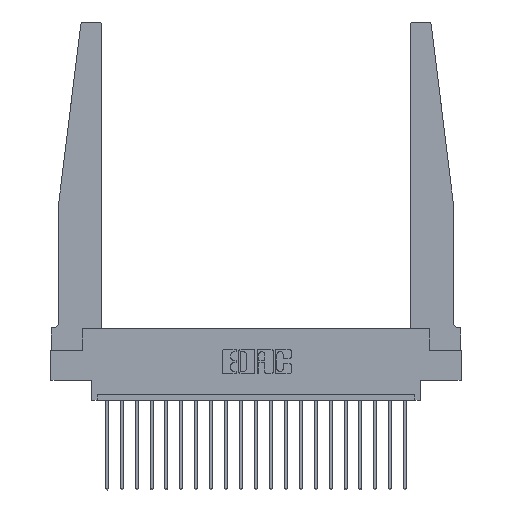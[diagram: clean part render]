
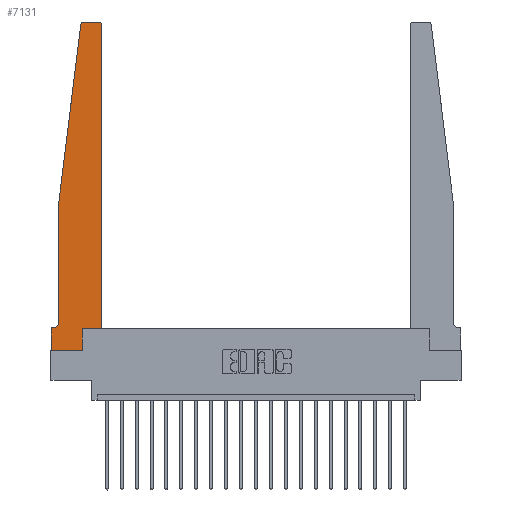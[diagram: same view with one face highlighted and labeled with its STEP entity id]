
A CAD part, top view. The second image highlights one B-rep face of the part: STEP entity #7131.
In plain terms, the highlighted planar face has unit normal (0, 0, 1).
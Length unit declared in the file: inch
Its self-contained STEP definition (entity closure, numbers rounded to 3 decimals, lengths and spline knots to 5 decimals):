
#42 = VECTOR ( 'NONE', #8179, 39.37008 ) ;
#329 = LINE ( 'NONE', #2886, #16862 ) ;
#640 = CARTESIAN_POINT ( 'NONE',  ( 0.27653, 2.75, 0.37 ) ) ;
#908 = CARTESIAN_POINT ( 'NONE',  ( 0.2605, 0.18, 0.37 ) ) ;
#1044 = ORIENTED_EDGE ( 'NONE', *, *, #4860, .T. ) ;
#1061 = DIRECTION ( 'NONE',  ( 0., 0., 1. ) ) ;
#1256 = VERTEX_POINT ( 'NONE', #11830 ) ;
#1284 = VERTEX_POINT ( 'NONE', #15466 ) ;
#1334 = DIRECTION ( 'NONE',  ( 0., 0., -1. ) ) ;
#1591 = CARTESIAN_POINT ( 'NONE',  ( 0.425, 0.18, 0.37 ) ) ;
#1922 = VECTOR ( 'NONE', #6121, 39.37008 ) ;
#2094 = CIRCLE ( 'NONE', #14696, 0.03 ) ;
#2648 = CARTESIAN_POINT ( 'NONE',  ( 0.395, 2.75, 0.37 ) ) ;
#2691 = DIRECTION ( 'NONE',  ( -1., 0., 0. ) ) ;
#2886 = CARTESIAN_POINT ( 'NONE',  ( 0.425, 0.18, 0.37 ) ) ;
#3394 = DIRECTION ( 'NONE',  ( 0., 0., 1. ) ) ;
#3483 = EDGE_CURVE ( 'NONE', #14115, #4005, #6902, .T. ) ;
#3516 = LINE ( 'NONE', #5672, #9023 ) ;
#3577 = FACE_OUTER_BOUND ( 'NONE', #15233, .T. ) ;
#4005 = VERTEX_POINT ( 'NONE', #640 ) ;
#4260 = DIRECTION ( 'NONE',  ( -1., 0., 0. ) ) ;
#4605 = EDGE_CURVE ( 'NONE', #6205, #5960, #329, .T. ) ;
#4860 = EDGE_CURVE ( 'NONE', #5960, #14115, #2094, .T. ) ;
#4876 = CARTESIAN_POINT ( 'NONE',  ( 0.27653, 2.72, 0.37 ) ) ;
#5551 = EDGE_CURVE ( 'NONE', #1284, #20755, #17089, .T. ) ;
#5671 = EDGE_CURVE ( 'NONE', #1256, #15966, #12101, .T. ) ;
#5672 = CARTESIAN_POINT ( 'NONE',  ( 0., 0., 0.37 ) ) ;
#5826 = EDGE_CURVE ( 'NONE', #4005, #1284, #11844, .T. ) ;
#5905 = ORIENTED_EDGE ( 'NONE', *, *, #5671, .T. ) ;
#5960 = VERTEX_POINT ( 'NONE', #11725 ) ;
#6121 = DIRECTION ( 'NONE',  ( 1., 0., 0. ) ) ;
#6205 = VERTEX_POINT ( 'NONE', #7276 ) ;
#6884 = DIRECTION ( 'NONE',  ( 0., 0., 1. ) ) ;
#6890 = DIRECTION ( 'NONE',  ( 0., 1., 0. ) ) ;
#6902 = LINE ( 'NONE', #16911, #10949 ) ;
#6997 = ORIENTED_EDGE ( 'NONE', *, *, #5551, .T. ) ;
#7131 = ADVANCED_FACE ( 'NONE', ( #3577 ), #10405, .T. ) ;
#7273 = CARTESIAN_POINT ( 'NONE',  ( 0.2605, 0., 0.37 ) ) ;
#7276 = CARTESIAN_POINT ( 'NONE',  ( 0.425, 0.18, 0.37 ) ) ;
#7565 = VECTOR ( 'NONE', #12845, 39.37008 ) ;
#7809 = EDGE_CURVE ( 'NONE', #20755, #13291, #15121, .T. ) ;
#8127 = CARTESIAN_POINT ( 'NONE',  ( 0.065, 1.25, 0.37 ) ) ;
#8179 = DIRECTION ( 'NONE',  ( -0.122, -0.992, 0. ) ) ;
#8331 = CARTESIAN_POINT ( 'NONE',  ( 0.065, 1.25, 0.37 ) ) ;
#9023 = VECTOR ( 'NONE', #12078, 39.37008 ) ;
#9513 = ORIENTED_EDGE ( 'NONE', *, *, #19324, .T. ) ;
#9873 = VERTEX_POINT ( 'NONE', #14425 ) ;
#10405 = PLANE ( 'NONE',  #18043 ) ;
#10487 = VECTOR ( 'NONE', #6890, 39.37008 ) ;
#10492 = LINE ( 'NONE', #17233, #17969 ) ;
#10684 = AXIS2_PLACEMENT_3D ( 'NONE', #4876, #3394, #11198 ) ;
#10885 = EDGE_CURVE ( 'NONE', #14520, #9873, #10492, .T. ) ;
#10949 = VECTOR ( 'NONE', #4260, 39.37008 ) ;
#11198 = DIRECTION ( 'NONE',  ( 1., 0., 0. ) ) ;
#11725 = CARTESIAN_POINT ( 'NONE',  ( 0.425, 2.72, 0.37 ) ) ;
#11830 = CARTESIAN_POINT ( 'NONE',  ( 0., 0., 0.37 ) ) ;
#11844 = CIRCLE ( 'NONE', #10684, 0.03 ) ;
#12078 = DIRECTION ( 'NONE',  ( 0., -1., 0. ) ) ;
#12101 = LINE ( 'NONE', #12699, #7565 ) ;
#12557 = DIRECTION ( 'NONE',  ( -1., 0., 0. ) ) ;
#12597 = VECTOR ( 'NONE', #14299, 39.37008 ) ;
#12699 = CARTESIAN_POINT ( 'NONE',  ( 0., 0., 0.37 ) ) ;
#12845 = DIRECTION ( 'NONE',  ( 1., 0., 0. ) ) ;
#12896 = CARTESIAN_POINT ( 'NONE',  ( 0.065, 1.25, 0.37 ) ) ;
#12916 = ORIENTED_EDGE ( 'NONE', *, *, #4605, .T. ) ;
#13291 = VERTEX_POINT ( 'NONE', #16721 ) ;
#13296 = VERTEX_POINT ( 'NONE', #908 ) ;
#13532 = EDGE_CURVE ( 'NONE', #13291, #14520, #18362, .T. ) ;
#13552 = CARTESIAN_POINT ( 'NONE',  ( 0.2605, 0.18, 0.37 ) ) ;
#13584 = AXIS2_PLACEMENT_3D ( 'NONE', #15706, #1334, #12557 ) ;
#13608 = CARTESIAN_POINT ( 'NONE',  ( 0.395, 2.72, 0.37 ) ) ;
#14115 = VERTEX_POINT ( 'NONE', #2648 ) ;
#14256 = EDGE_CURVE ( 'NONE', #13296, #6205, #14448, .T. ) ;
#14299 = DIRECTION ( 'NONE',  ( 0., -1., 0. ) ) ;
#14425 = CARTESIAN_POINT ( 'NONE',  ( 0., 0.1875, 0.37 ) ) ;
#14448 = LINE ( 'NONE', #1591, #1922 ) ;
#14496 = ORIENTED_EDGE ( 'NONE', *, *, #5826, .T. ) ;
#14520 = VERTEX_POINT ( 'NONE', #18617 ) ;
#14696 = AXIS2_PLACEMENT_3D ( 'NONE', #13608, #1061, #19962 ) ;
#15121 = LINE ( 'NONE', #8127, #12597 ) ;
#15233 = EDGE_LOOP ( 'NONE', ( #17703, #14496, #6997, #20612, #19481, #15245, #16713, #5905, #9513, #16724, #12916, #1044 ) ) ;
#15245 = ORIENTED_EDGE ( 'NONE', *, *, #10885, .T. ) ;
#15466 = CARTESIAN_POINT ( 'NONE',  ( 0.24675, 2.72367, 0.37 ) ) ;
#15706 = CARTESIAN_POINT ( 'NONE',  ( 0.015, 0.2375, 0.37 ) ) ;
#15966 = VERTEX_POINT ( 'NONE', #7273 ) ;
#16473 = CARTESIAN_POINT ( 'NONE',  ( 0., 0.1875, 0.37 ) ) ;
#16713 = ORIENTED_EDGE ( 'NONE', *, *, #18100, .T. ) ;
#16721 = CARTESIAN_POINT ( 'NONE',  ( 0.065, 0.2375, 0.37 ) ) ;
#16724 = ORIENTED_EDGE ( 'NONE', *, *, #14256, .T. ) ;
#16862 = VECTOR ( 'NONE', #18879, 39.37008 ) ;
#16911 = CARTESIAN_POINT ( 'NONE',  ( 0.25, 2.75, 0.37 ) ) ;
#17089 = LINE ( 'NONE', #12896, #42 ) ;
#17233 = CARTESIAN_POINT ( 'NONE',  ( 0.065, 0.1875, 0.37 ) ) ;
#17703 = ORIENTED_EDGE ( 'NONE', *, *, #3483, .T. ) ;
#17969 = VECTOR ( 'NONE', #2691, 39.37008 ) ;
#18043 = AXIS2_PLACEMENT_3D ( 'NONE', #16473, #6884, #19684 ) ;
#18100 = EDGE_CURVE ( 'NONE', #9873, #1256, #3516, .T. ) ;
#18362 = CIRCLE ( 'NONE', #13584, 0.05 ) ;
#18617 = CARTESIAN_POINT ( 'NONE',  ( 0.015, 0.1875, 0.37 ) ) ;
#18879 = DIRECTION ( 'NONE',  ( 0., 1., 0. ) ) ;
#19324 = EDGE_CURVE ( 'NONE', #15966, #13296, #19703, .T. ) ;
#19481 = ORIENTED_EDGE ( 'NONE', *, *, #13532, .T. ) ;
#19684 = DIRECTION ( 'NONE',  ( 1., 0., 0. ) ) ;
#19703 = LINE ( 'NONE', #13552, #10487 ) ;
#19962 = DIRECTION ( 'NONE',  ( 1., 0., 0. ) ) ;
#20612 = ORIENTED_EDGE ( 'NONE', *, *, #7809, .T. ) ;
#20755 = VERTEX_POINT ( 'NONE', #8331 ) ;
